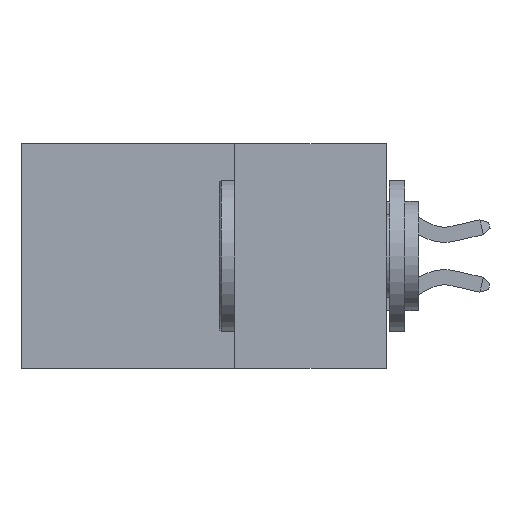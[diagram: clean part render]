
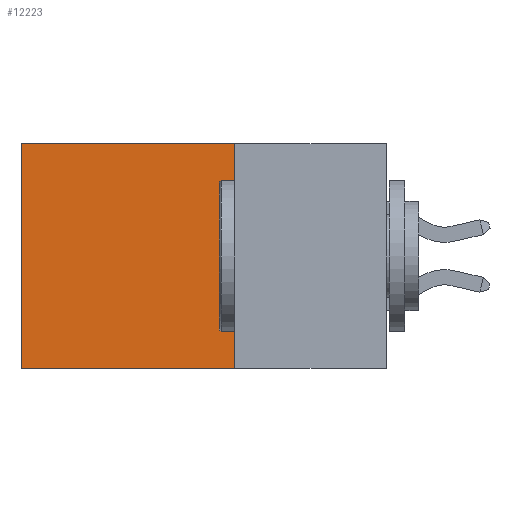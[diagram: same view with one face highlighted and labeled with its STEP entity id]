
A CAD part, left-side view. The second image highlights one B-rep face of the part: STEP entity #12223.
In plain terms, the highlighted planar face has unit normal (-1, 0, 0).
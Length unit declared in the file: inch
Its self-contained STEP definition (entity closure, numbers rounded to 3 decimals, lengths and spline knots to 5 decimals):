
#252 = CARTESIAN_POINT ( 'NONE',  ( 0.2615, 0.6, -0.37 ) ) ;
#389 = CARTESIAN_POINT ( 'NONE',  ( 0.2615, 0.25, -0.37 ) ) ;
#1026 = EDGE_CURVE ( 'NONE', #14136, #12125, #4658, .T. ) ;
#1122 = VECTOR ( 'NONE', #13531, 39.37008 ) ;
#1172 = ORIENTED_EDGE ( 'NONE', *, *, #6194, .F. ) ;
#1390 = ORIENTED_EDGE ( 'NONE', *, *, #6086, .T. ) ;
#2674 = LINE ( 'NONE', #7806, #12330 ) ;
#3299 = PLANE ( 'NONE',  #5944 ) ;
#4407 = VECTOR ( 'NONE', #6946, 39.37008 ) ;
#4516 = DIRECTION ( 'NONE',  ( 1., 0., 0. ) ) ;
#4658 = LINE ( 'NONE', #9389, #4407 ) ;
#4800 = CARTESIAN_POINT ( 'NONE',  ( 0.2615, 0.25, 0. ) ) ;
#5325 = CARTESIAN_POINT ( 'NONE',  ( 0.2615, 0.6, 0. ) ) ;
#5944 = AXIS2_PLACEMENT_3D ( 'NONE', #10724, #4516, #15924 ) ;
#6086 = EDGE_CURVE ( 'NONE', #14136, #9766, #11087, .T. ) ;
#6194 = EDGE_CURVE ( 'NONE', #12125, #14950, #2674, .T. ) ;
#6946 = DIRECTION ( 'NONE',  ( 0., 0., -1. ) ) ;
#7806 = CARTESIAN_POINT ( 'NONE',  ( 0.2615, 0.25, -0.37 ) ) ;
#8080 = ORIENTED_EDGE ( 'NONE', *, *, #8484, .T. ) ;
#8484 = EDGE_CURVE ( 'NONE', #9766, #14950, #13969, .T. ) ;
#8865 = DIRECTION ( 'NONE',  ( 0., 1., 0. ) ) ;
#9334 = CARTESIAN_POINT ( 'NONE',  ( 0.2615, 0.25, 0. ) ) ;
#9389 = CARTESIAN_POINT ( 'NONE',  ( 0.2615, 0.25, -0.37 ) ) ;
#9766 = VERTEX_POINT ( 'NONE', #5325 ) ;
#9900 = EDGE_LOOP ( 'NONE', ( #8080, #1172, #13772, #1390 ) ) ;
#10724 = CARTESIAN_POINT ( 'NONE',  ( 0.2615, 0.25, -0.37 ) ) ;
#10959 = FACE_OUTER_BOUND ( 'NONE', #9900, .T. ) ;
#11073 = VECTOR ( 'NONE', #12677, 39.37008 ) ;
#11087 = LINE ( 'NONE', #4800, #1122 ) ;
#12125 = VERTEX_POINT ( 'NONE', #389 ) ;
#12223 = ADVANCED_FACE ( 'NONE', ( #10959 ), #3299, .F. ) ;
#12330 = VECTOR ( 'NONE', #8865, 39.37008 ) ;
#12677 = DIRECTION ( 'NONE',  ( 0., 0., -1. ) ) ;
#13531 = DIRECTION ( 'NONE',  ( 0., 1., 0. ) ) ;
#13772 = ORIENTED_EDGE ( 'NONE', *, *, #1026, .F. ) ;
#13969 = LINE ( 'NONE', #14959, #11073 ) ;
#14136 = VERTEX_POINT ( 'NONE', #9334 ) ;
#14950 = VERTEX_POINT ( 'NONE', #252 ) ;
#14959 = CARTESIAN_POINT ( 'NONE',  ( 0.2615, 0.6, -0.37 ) ) ;
#15924 = DIRECTION ( 'NONE',  ( 0., 0., -1. ) ) ;
